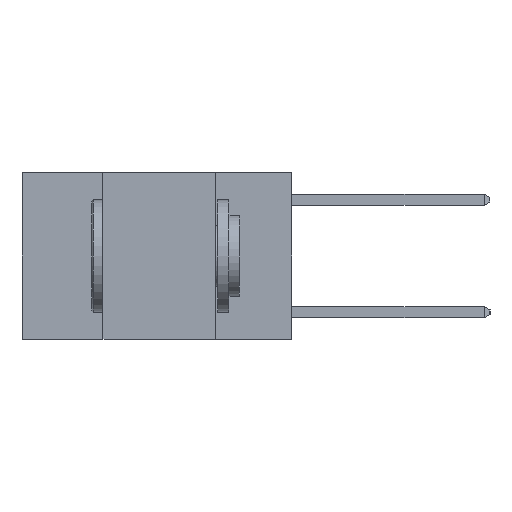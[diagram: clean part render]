
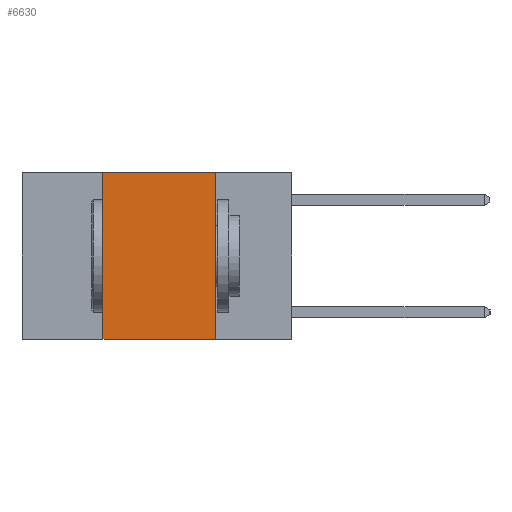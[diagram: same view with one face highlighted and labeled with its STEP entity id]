
A CAD part, left-side view. The second image highlights one B-rep face of the part: STEP entity #6630.
In plain terms, the highlighted planar face has unit normal (-1, 0, 0).
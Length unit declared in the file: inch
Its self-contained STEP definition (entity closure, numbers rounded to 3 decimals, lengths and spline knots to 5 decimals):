
#255 = VECTOR ( 'NONE', #1074, 39.37008 ) ;
#281 = DIRECTION ( 'NONE',  ( 0., 0., 1. ) ) ;
#341 = CARTESIAN_POINT ( 'NONE',  ( 0., 0.6, -0.37 ) ) ;
#507 = CARTESIAN_POINT ( 'NONE',  ( 0., 0.42, 0. ) ) ;
#569 = DIRECTION ( 'NONE',  ( 0., 0., -1. ) ) ;
#834 = ORIENTED_EDGE ( 'NONE', *, *, #1818, .F. ) ;
#1074 = DIRECTION ( 'NONE',  ( 0., -1., 0. ) ) ;
#1326 = CARTESIAN_POINT ( 'NONE',  ( 0., 0.17, 0. ) ) ;
#1746 = EDGE_CURVE ( 'NONE', #3088, #5730, #6083, .T. ) ;
#1759 = ORIENTED_EDGE ( 'NONE', *, *, #1746, .F. ) ;
#1818 = EDGE_CURVE ( 'NONE', #5730, #6887, #5624, .T. ) ;
#2799 = PLANE ( 'NONE',  #7900 ) ;
#2934 = CARTESIAN_POINT ( 'NONE',  ( 0., 0.6, 0. ) ) ;
#2944 = EDGE_CURVE ( 'NONE', #3088, #7614, #7744, .T. ) ;
#3002 = DIRECTION ( 'NONE',  ( 0., -1., 0. ) ) ;
#3088 = VERTEX_POINT ( 'NONE', #6332 ) ;
#3207 = CARTESIAN_POINT ( 'NONE',  ( 0., 0.42, 0. ) ) ;
#3361 = ORIENTED_EDGE ( 'NONE', *, *, #2944, .T. ) ;
#3556 = DIRECTION ( 'NONE',  ( 0., 0., -1. ) ) ;
#3602 = FACE_OUTER_BOUND ( 'NONE', #6249, .T. ) ;
#3936 = VECTOR ( 'NONE', #569, 39.37008 ) ;
#4989 = CARTESIAN_POINT ( 'NONE',  ( 0., 0.6, 0. ) ) ;
#5412 = CARTESIAN_POINT ( 'NONE',  ( 0., 0.17, -0.37 ) ) ;
#5624 = LINE ( 'NONE', #2934, #7306 ) ;
#5730 = VERTEX_POINT ( 'NONE', #3207 ) ;
#6083 = LINE ( 'NONE', #507, #8217 ) ;
#6249 = EDGE_LOOP ( 'NONE', ( #8787, #834, #1759, #3361 ) ) ;
#6332 = CARTESIAN_POINT ( 'NONE',  ( 0., 0.42, -0.37 ) ) ;
#6630 = ADVANCED_FACE ( 'NONE', ( #3602 ), #2799, .F. ) ;
#6887 = VERTEX_POINT ( 'NONE', #7476 ) ;
#7199 = EDGE_CURVE ( 'NONE', #6887, #7614, #7777, .T. ) ;
#7306 = VECTOR ( 'NONE', #3002, 39.37008 ) ;
#7476 = CARTESIAN_POINT ( 'NONE',  ( 0., 0.17, 0. ) ) ;
#7614 = VERTEX_POINT ( 'NONE', #5412 ) ;
#7744 = LINE ( 'NONE', #341, #255 ) ;
#7777 = LINE ( 'NONE', #1326, #3936 ) ;
#7886 = DIRECTION ( 'NONE',  ( 1., 0., 0. ) ) ;
#7900 = AXIS2_PLACEMENT_3D ( 'NONE', #4989, #7886, #3556 ) ;
#8217 = VECTOR ( 'NONE', #281, 39.37008 ) ;
#8787 = ORIENTED_EDGE ( 'NONE', *, *, #7199, .F. ) ;
